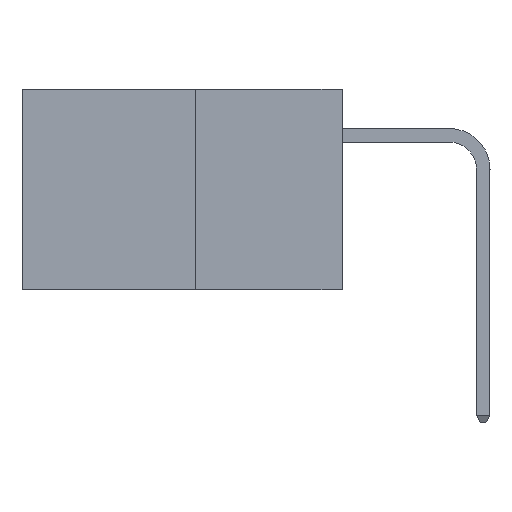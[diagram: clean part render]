
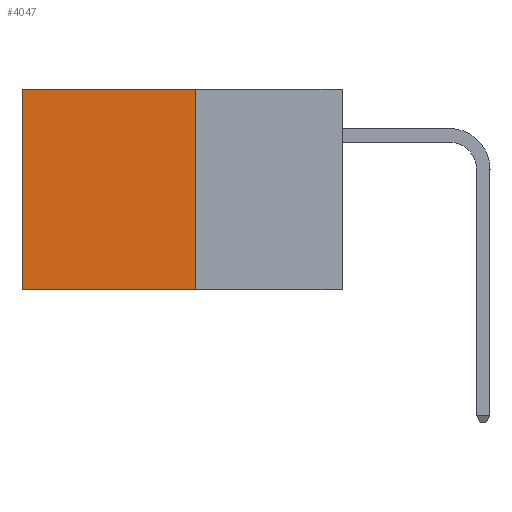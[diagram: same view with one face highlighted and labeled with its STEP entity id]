
A CAD part, left-side view. The second image highlights one B-rep face of the part: STEP entity #4047.
In plain terms, the highlighted planar face has unit normal (-1, 0, 0).
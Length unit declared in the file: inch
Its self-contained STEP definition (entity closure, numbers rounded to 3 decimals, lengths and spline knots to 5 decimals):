
#141 = VERTEX_POINT ( 'NONE', #1994 ) ;
#1050 = VECTOR ( 'NONE', #6154, 39.37008 ) ;
#1104 = VECTOR ( 'NONE', #10482, 39.37008 ) ;
#1165 = CARTESIAN_POINT ( 'NONE',  ( 0.277, 0.27, 0. ) ) ;
#1466 = PLANE ( 'NONE',  #6747 ) ;
#1994 = CARTESIAN_POINT ( 'NONE',  ( 0.277, 0.27, -0.37 ) ) ;
#2058 = LINE ( 'NONE', #8004, #12547 ) ;
#2162 = ORIENTED_EDGE ( 'NONE', *, *, #2349, .T. ) ;
#2349 = EDGE_CURVE ( 'NONE', #9116, #10393, #9016, .T. ) ;
#2775 = CARTESIAN_POINT ( 'NONE',  ( 0.277, 0.59, 0. ) ) ;
#2792 = DIRECTION ( 'NONE',  ( 1., 0., 0. ) ) ;
#3818 = LINE ( 'NONE', #6515, #1050 ) ;
#4047 = ADVANCED_FACE ( 'NONE', ( #12559 ), #1466, .F. ) ;
#4400 = CARTESIAN_POINT ( 'NONE',  ( 0.277, 0.27, -0.37 ) ) ;
#4437 = EDGE_CURVE ( 'NONE', #9116, #141, #2058, .T. ) ;
#4540 = VERTEX_POINT ( 'NONE', #12823 ) ;
#4573 = ORIENTED_EDGE ( 'NONE', *, *, #4437, .F. ) ;
#6154 = DIRECTION ( 'NONE',  ( 0., 0., -1. ) ) ;
#6515 = CARTESIAN_POINT ( 'NONE',  ( 0.277, 0.59, -0.37 ) ) ;
#6600 = LINE ( 'NONE', #4400, #1104 ) ;
#6634 = VECTOR ( 'NONE', #9305, 39.37008 ) ;
#6747 = AXIS2_PLACEMENT_3D ( 'NONE', #7283, #2792, #12488 ) ;
#7283 = CARTESIAN_POINT ( 'NONE',  ( 0.277, 0.27, -0.37 ) ) ;
#7658 = CARTESIAN_POINT ( 'NONE',  ( 0.277, 0.27, 0. ) ) ;
#8004 = CARTESIAN_POINT ( 'NONE',  ( 0.277, 0.27, -0.37 ) ) ;
#9016 = LINE ( 'NONE', #7658, #6634 ) ;
#9116 = VERTEX_POINT ( 'NONE', #1165 ) ;
#9305 = DIRECTION ( 'NONE',  ( 0., 1., 0. ) ) ;
#10222 = EDGE_CURVE ( 'NONE', #10393, #4540, #3818, .T. ) ;
#10295 = DIRECTION ( 'NONE',  ( 0., 0., -1. ) ) ;
#10393 = VERTEX_POINT ( 'NONE', #2775 ) ;
#10482 = DIRECTION ( 'NONE',  ( 0., 1., 0. ) ) ;
#11351 = EDGE_CURVE ( 'NONE', #141, #4540, #6600, .T. ) ;
#11449 = EDGE_LOOP ( 'NONE', ( #12034, #12338, #4573, #2162 ) ) ;
#12034 = ORIENTED_EDGE ( 'NONE', *, *, #10222, .T. ) ;
#12338 = ORIENTED_EDGE ( 'NONE', *, *, #11351, .F. ) ;
#12488 = DIRECTION ( 'NONE',  ( 0., 0., -1. ) ) ;
#12547 = VECTOR ( 'NONE', #10295, 39.37008 ) ;
#12559 = FACE_OUTER_BOUND ( 'NONE', #11449, .T. ) ;
#12823 = CARTESIAN_POINT ( 'NONE',  ( 0.277, 0.59, -0.37 ) ) ;
